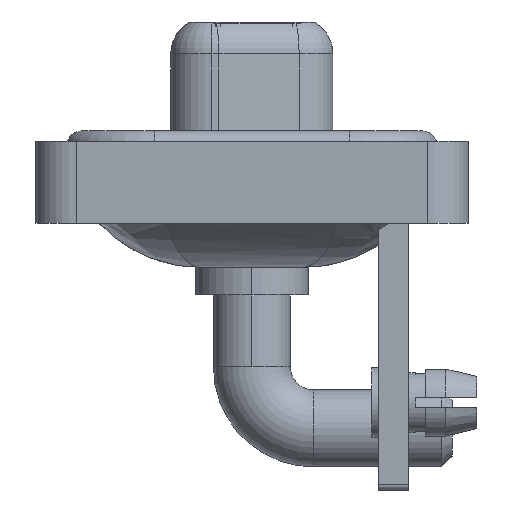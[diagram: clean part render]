
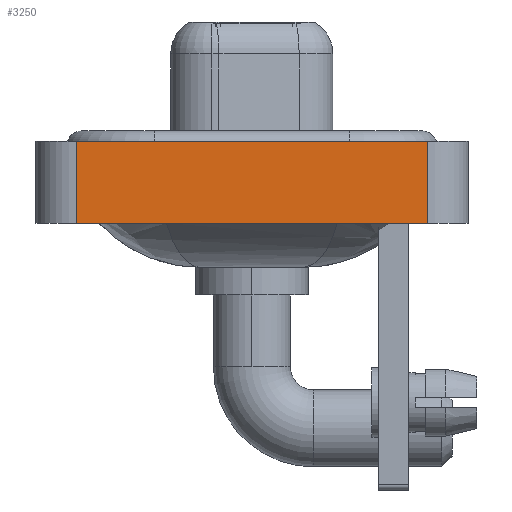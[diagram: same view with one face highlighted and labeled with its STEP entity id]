
A CAD part, left-side view. The second image highlights one B-rep face of the part: STEP entity #3250.
In plain terms, the highlighted planar face has unit normal (-1, 0, 0).
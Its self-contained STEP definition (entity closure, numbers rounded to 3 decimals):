
#465 = CARTESIAN_POINT ( 'NONE',  ( -7.35, -8.55, -3.6 ) ) ;
#1442 = EDGE_CURVE ( 'NONE', #12263, #13645, #18153, .T. ) ;
#2176 = VECTOR ( 'NONE', #10161, 1000. ) ;
#2956 = ORIENTED_EDGE ( 'NONE', *, *, #14787, .F. ) ;
#3137 = ORIENTED_EDGE ( 'NONE', *, *, #1442, .T. ) ;
#3250 = ADVANCED_FACE ( 'NONE', ( #11618 ), #12887, .T. ) ;
#3290 = ORIENTED_EDGE ( 'NONE', *, *, #12787, .F. ) ;
#4347 = CARTESIAN_POINT ( 'NONE',  ( -7.35, -8.55, -3.6 ) ) ;
#5586 = DIRECTION ( 'NONE',  ( -1., 0., 0. ) ) ;
#5776 = EDGE_LOOP ( 'NONE', ( #17972, #3290, #2956, #3137 ) ) ;
#6001 = CARTESIAN_POINT ( 'NONE',  ( -7.35, 8.55, 0.4 ) ) ;
#6184 = LINE ( 'NONE', #17891, #7849 ) ;
#6280 = DIRECTION ( 'NONE',  ( 0., 0., 1. ) ) ;
#7440 = CARTESIAN_POINT ( 'NONE',  ( -7.35, -8.55, 0.4 ) ) ;
#7820 = DIRECTION ( 'NONE',  ( 0., 0., 1. ) ) ;
#7849 = VECTOR ( 'NONE', #6280, 1000. ) ;
#8111 = CARTESIAN_POINT ( 'NONE',  ( -7.35, -8.55, -3.6 ) ) ;
#9445 = EDGE_CURVE ( 'NONE', #13645, #14613, #14070, .T. ) ;
#10007 = CARTESIAN_POINT ( 'NONE',  ( -7.35, -8.55, -3.6 ) ) ;
#10161 = DIRECTION ( 'NONE',  ( 0., -1., 0. ) ) ;
#11618 = FACE_OUTER_BOUND ( 'NONE', #5776, .T. ) ;
#12263 = VERTEX_POINT ( 'NONE', #14579 ) ;
#12787 = EDGE_CURVE ( 'NONE', #14670, #14613, #14856, .T. ) ;
#12887 = PLANE ( 'NONE',  #16039 ) ;
#13131 = CARTESIAN_POINT ( 'NONE',  ( -7.35, -8.55, 0.4 ) ) ;
#13645 = VERTEX_POINT ( 'NONE', #4347 ) ;
#13672 = DIRECTION ( 'NONE',  ( 0., -1., 0. ) ) ;
#14070 = LINE ( 'NONE', #8111, #16670 ) ;
#14579 = CARTESIAN_POINT ( 'NONE',  ( -7.35, 8.55, -3.6 ) ) ;
#14613 = VERTEX_POINT ( 'NONE', #7440 ) ;
#14670 = VERTEX_POINT ( 'NONE', #6001 ) ;
#14787 = EDGE_CURVE ( 'NONE', #12263, #14670, #6184, .T. ) ;
#14856 = LINE ( 'NONE', #13131, #2176 ) ;
#15745 = VECTOR ( 'NONE', #13672, 1000. ) ;
#16039 = AXIS2_PLACEMENT_3D ( 'NONE', #10007, #5586, #17458 ) ;
#16670 = VECTOR ( 'NONE', #7820, 1000. ) ;
#17458 = DIRECTION ( 'NONE',  ( 0., 0., 1. ) ) ;
#17891 = CARTESIAN_POINT ( 'NONE',  ( -7.35, 8.55, -3.6 ) ) ;
#17972 = ORIENTED_EDGE ( 'NONE', *, *, #9445, .T. ) ;
#18153 = LINE ( 'NONE', #465, #15745 ) ;
